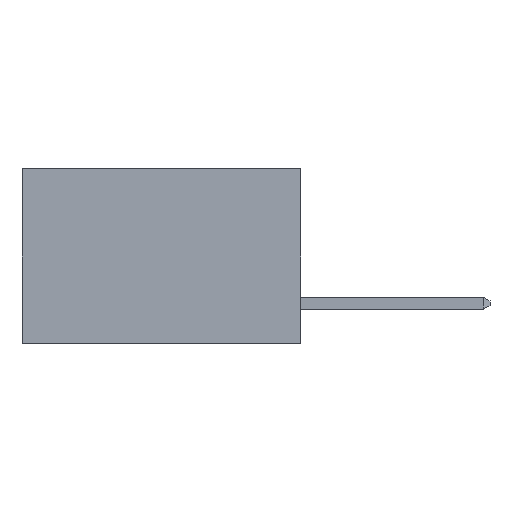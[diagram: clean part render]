
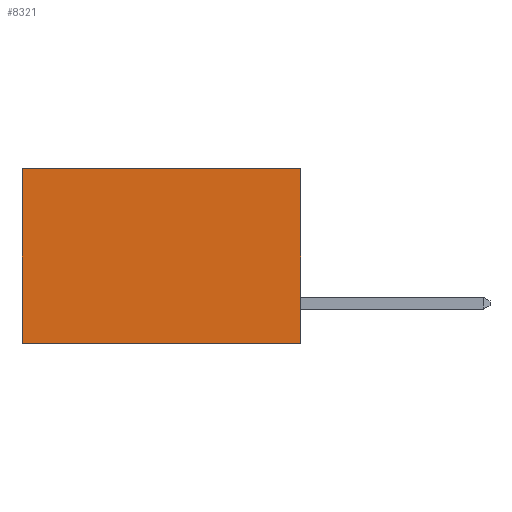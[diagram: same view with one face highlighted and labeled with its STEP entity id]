
A CAD part, left-side view. The second image highlights one B-rep face of the part: STEP entity #8321.
In plain terms, the highlighted planar face has unit normal (-1, 0, 0).
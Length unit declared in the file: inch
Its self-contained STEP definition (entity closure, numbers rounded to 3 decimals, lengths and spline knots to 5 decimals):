
#370 = EDGE_LOOP ( 'NONE', ( #2523, #2538, #2559, #2691 ) ) ;
#660 = LINE ( 'NONE', #4395, #8580 ) ;
#708 = VECTOR ( 'NONE', #4283, 39.37008 ) ;
#804 = EDGE_CURVE ( 'NONE', #2082, #6564, #4515, .T. ) ;
#902 = PLANE ( 'NONE',  #7451 ) ;
#907 = CARTESIAN_POINT ( 'NONE',  ( 0.277, 0.59, 0. ) ) ;
#1029 = CARTESIAN_POINT ( 'NONE',  ( 0.277, 0.59, -0.37 ) ) ;
#1723 = DIRECTION ( 'NONE',  ( 1., 0., 0. ) ) ;
#2082 = VERTEX_POINT ( 'NONE', #3699 ) ;
#2523 = ORIENTED_EDGE ( 'NONE', *, *, #3506, .T. ) ;
#2538 = ORIENTED_EDGE ( 'NONE', *, *, #804, .F. ) ;
#2559 = ORIENTED_EDGE ( 'NONE', *, *, #7180, .F. ) ;
#2691 = ORIENTED_EDGE ( 'NONE', *, *, #7067, .T. ) ;
#2980 = VERTEX_POINT ( 'NONE', #7480 ) ;
#3506 = EDGE_CURVE ( 'NONE', #4545, #6564, #660, .T. ) ;
#3699 = CARTESIAN_POINT ( 'NONE',  ( 0.277, 0., -0.37 ) ) ;
#3757 = CARTESIAN_POINT ( 'NONE',  ( 0.277, 0., -0.37 ) ) ;
#4014 = LINE ( 'NONE', #5856, #7672 ) ;
#4021 = VECTOR ( 'NONE', #8394, 39.37008 ) ;
#4283 = DIRECTION ( 'NONE',  ( 0., 1., 0. ) ) ;
#4395 = CARTESIAN_POINT ( 'NONE',  ( 0.277, 0.59, -0.37 ) ) ;
#4515 = LINE ( 'NONE', #3757, #4021 ) ;
#4545 = VERTEX_POINT ( 'NONE', #907 ) ;
#4774 = FACE_OUTER_BOUND ( 'NONE', #370, .T. ) ;
#5024 = CARTESIAN_POINT ( 'NONE',  ( 0.277, 0., 0. ) ) ;
#5197 = LINE ( 'NONE', #5024, #708 ) ;
#5856 = CARTESIAN_POINT ( 'NONE',  ( 0.277, 0., -0.37 ) ) ;
#6337 = CARTESIAN_POINT ( 'NONE',  ( 0.277, 0., -0.37 ) ) ;
#6564 = VERTEX_POINT ( 'NONE', #1029 ) ;
#7033 = DIRECTION ( 'NONE',  ( 0., 0., -1. ) ) ;
#7067 = EDGE_CURVE ( 'NONE', #2980, #4545, #5197, .T. ) ;
#7180 = EDGE_CURVE ( 'NONE', #2980, #2082, #4014, .T. ) ;
#7291 = DIRECTION ( 'NONE',  ( 0., 0., -1. ) ) ;
#7451 = AXIS2_PLACEMENT_3D ( 'NONE', #6337, #1723, #7033 ) ;
#7480 = CARTESIAN_POINT ( 'NONE',  ( 0.277, 0., 0. ) ) ;
#7672 = VECTOR ( 'NONE', #7291, 39.37008 ) ;
#8321 = ADVANCED_FACE ( 'NONE', ( #4774 ), #902, .F. ) ;
#8394 = DIRECTION ( 'NONE',  ( 0., 1., 0. ) ) ;
#8580 = VECTOR ( 'NONE', #8737, 39.37008 ) ;
#8737 = DIRECTION ( 'NONE',  ( 0., 0., -1. ) ) ;
